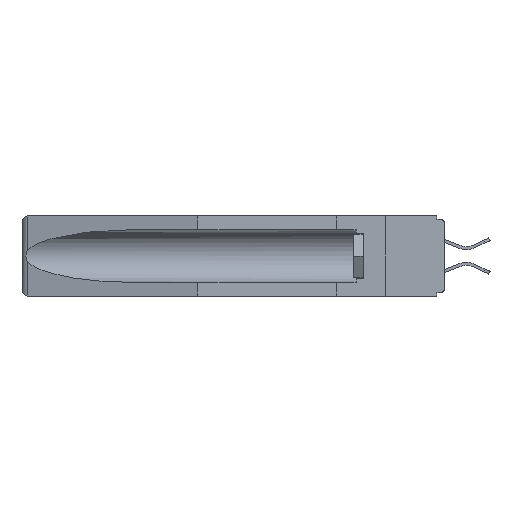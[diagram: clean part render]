
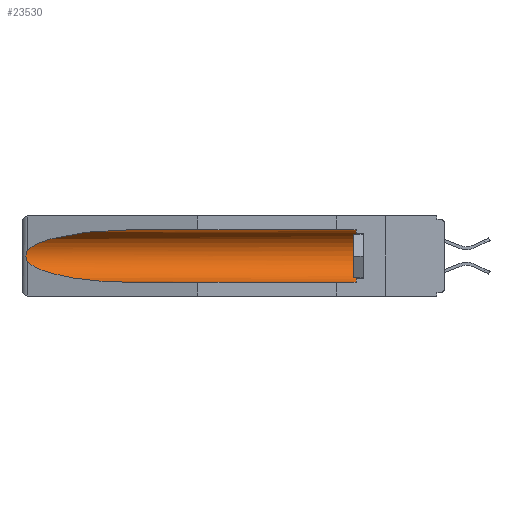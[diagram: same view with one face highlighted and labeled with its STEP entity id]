
A CAD part, left-side view. The second image highlights one B-rep face of the part: STEP entity #23530.
In plain terms, the highlighted cylindrical face has radius 2.857 mm (diameter 5.715 mm), a partial arc.
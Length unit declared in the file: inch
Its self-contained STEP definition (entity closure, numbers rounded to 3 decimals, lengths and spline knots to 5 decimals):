
#52 = DIRECTION ( 'NONE',  ( 0., 0., 1. ) ) ;
#1085 = VERTEX_POINT ( 'NONE', #6895 ) ;
#1866 = CARTESIAN_POINT ( 'NONE',  ( 0.155, 1.07973, -0.059 ) ) ;
#2327 = CARTESIAN_POINT ( 'NONE',  ( 0.2675, 1.53308, -0.17534 ) ) ;
#3081 = CARTESIAN_POINT ( 'NONE',  ( 0.26537, 1.52718, -0.14972 ) ) ;
#4478 = CARTESIAN_POINT ( 'NONE',  ( 0.21114, 1.30732, -0.059 ) ) ;
#4778 = LINE ( 'NONE', #22943, #26740 ) ;
#5231 = ORIENTED_EDGE ( 'NONE', *, *, #8693, .T. ) ;
#5910 = CARTESIAN_POINT ( 'NONE',  ( 0.26537, 1.52718, -0.14972 ) ) ;
#6361 = ORIENTED_EDGE ( 'NONE', *, *, #7550, .F. ) ;
#6895 = CARTESIAN_POINT ( 'NONE',  ( 0.155, 0.126, -0.284 ) ) ;
#7322 = DIRECTION ( 'NONE',  ( 0., -1., 0. ) ) ;
#7347 = CARTESIAN_POINT ( 'NONE',  ( 0.26537, 1.52718, -0.19328 ) ) ;
#7550 = EDGE_CURVE ( 'NONE', #1085, #33458, #25398, .T. ) ;
#8027 = CARTESIAN_POINT ( 'NONE',  ( 0.155, 1.07973, -0.284 ) ) ;
#8248 = CARTESIAN_POINT ( 'NONE',  ( 0.155, -0.30754, -0.1715 ) ) ;
#8582 = ORIENTED_EDGE ( 'NONE', *, *, #8944, .T. ) ;
#8693 = EDGE_CURVE ( 'NONE', #29670, #9239, #23338, .T. ) ;
#8930 = CARTESIAN_POINT ( 'NONE',  ( 0.21114, 1.30732, -0.284 ) ) ;
#8944 = EDGE_CURVE ( 'NONE', #17884, #33458, #21247, .T. ) ;
#9044 = CARTESIAN_POINT ( 'NONE',  ( 0.25451, 1.48313, -0.24835 ) ) ;
#9144 = EDGE_CURVE ( 'NONE', #1085, #13082, #14642, .T. ) ;
#9194 = B_SPLINE_CURVE_WITH_KNOTS ( 'NONE', 3,
 ( #25549, #17836, #28146, #22762, #15368, #2327, #33280, #22879, #20251, #7347 ),
 .UNSPECIFIED., .F., .F.,
 ( 4, 2, 2, 2, 4 ),
 ( 0., 0.00029, 0.00058, 0.00087, 0.00117 ),
 .UNSPECIFIED. ) ;
#9239 = VERTEX_POINT ( 'NONE', #5910 ) ;
#9697 = DIRECTION ( 'NONE',  ( 0., 1., 0. ) ) ;
#12210 = AXIS2_PLACEMENT_3D ( 'NONE', #14902, #7322, #28242 ) ;
#13082 = VERTEX_POINT ( 'NONE', #18282 ) ;
#13324 = CARTESIAN_POINT ( 'NONE',  ( 0.26537, 1.52718, -0.19328 ) ) ;
#13930 = EDGE_LOOP ( 'NONE', ( #5231, #24977, #8582, #6361, #14669, #17929 ) ) ;
#14642 = CIRCLE ( 'NONE', #12210, 0.1125 ) ;
#14669 = ORIENTED_EDGE ( 'NONE', *, *, #9144, .T. ) ;
#14902 = CARTESIAN_POINT ( 'NONE',  ( 0.155, 0.126, -0.1715 ) ) ;
#15368 = CARTESIAN_POINT ( 'NONE',  ( 0.2675, 1.53308, -0.16763 ) ) ;
#15626 = DIRECTION ( 'NONE',  ( 0., 1., 0. ) ) ;
#15859 = CARTESIAN_POINT ( 'NONE',  ( 0.155, -0.30754, -0.284 ) ) ;
#17167 = CARTESIAN_POINT ( 'NONE',  ( 0.155, 1.07973, -0.059 ) ) ;
#17569 = VECTOR ( 'NONE', #21223, 39.37008 ) ;
#17774 = CARTESIAN_POINT ( 'NONE',  ( 0.26537, 1.52718, -0.19328 ) ) ;
#17836 = CARTESIAN_POINT ( 'NONE',  ( 0.26597, 1.52961, -0.15275 ) ) ;
#17884 = VERTEX_POINT ( 'NONE', #17774 ) ;
#17929 = ORIENTED_EDGE ( 'NONE', *, *, #24945, .T. ) ;
#18029 = CARTESIAN_POINT ( 'NONE',  ( 0.25451, 1.48313, -0.09465 ) ) ;
#18282 = CARTESIAN_POINT ( 'NONE',  ( 0.155, 0.126, -0.059 ) ) ;
#19483 = CYLINDRICAL_SURFACE ( 'NONE', #28764, 0.1125 ) ;
#20251 = CARTESIAN_POINT ( 'NONE',  ( 0.26597, 1.5296, -0.19026 ) ) ;
#21171 = CARTESIAN_POINT ( 'NONE',  ( 0.155, 1.07973, -0.284 ) ) ;
#21223 = DIRECTION ( 'NONE',  ( 0., 1., 0. ) ) ;
#21247 =( BOUNDED_CURVE ( )  B_SPLINE_CURVE ( 3, ( #13324, #9044, #8930, #21171 ),
 .UNSPECIFIED., .F., .F. ) 
 B_SPLINE_CURVE_WITH_KNOTS ( ( 4, 4 ),
 ( 0.1948, 1.5708 ),
 .UNSPECIFIED. ) 
 CURVE ( )  GEOMETRIC_REPRESENTATION_ITEM ( )  RATIONAL_B_SPLINE_CURVE ( ( 1., 0.848, 0.848, 1. ) ) 
 REPRESENTATION_ITEM ( '' )  );
#22762 = CARTESIAN_POINT ( 'NONE',  ( 0.2673, 1.5327, -0.16383 ) ) ;
#22776 = FACE_OUTER_BOUND ( 'NONE', #13930, .T. ) ;
#22879 = CARTESIAN_POINT ( 'NONE',  ( 0.26655, 1.53094, -0.18657 ) ) ;
#22943 = CARTESIAN_POINT ( 'NONE',  ( 0.155, -0.30754, -0.059 ) ) ;
#23338 =( BOUNDED_CURVE ( )  B_SPLINE_CURVE ( 3, ( #1866, #4478, #18029, #3081 ),
 .UNSPECIFIED., .F., .F. ) 
 B_SPLINE_CURVE_WITH_KNOTS ( ( 4, 4 ),
 ( 4.71239, 6.08839 ),
 .UNSPECIFIED. ) 
 CURVE ( )  GEOMETRIC_REPRESENTATION_ITEM ( )  RATIONAL_B_SPLINE_CURVE ( ( 1., 0.848, 0.848, 1. ) ) 
 REPRESENTATION_ITEM ( '' )  );
#23530 = ADVANCED_FACE ( 'NONE', ( #22776 ), #19483, .F. ) ;
#24945 = EDGE_CURVE ( 'NONE', #13082, #29670, #4778, .T. ) ;
#24977 = ORIENTED_EDGE ( 'NONE', *, *, #28274, .T. ) ;
#25398 = LINE ( 'NONE', #15859, #17569 ) ;
#25549 = CARTESIAN_POINT ( 'NONE',  ( 0.26537, 1.52718, -0.14972 ) ) ;
#26740 = VECTOR ( 'NONE', #9697, 39.37008 ) ;
#28146 = CARTESIAN_POINT ( 'NONE',  ( 0.26654, 1.53092, -0.15636 ) ) ;
#28242 = DIRECTION ( 'NONE',  ( 0., 0., 1. ) ) ;
#28274 = EDGE_CURVE ( 'NONE', #9239, #17884, #9194, .T. ) ;
#28764 = AXIS2_PLACEMENT_3D ( 'NONE', #8248, #15626, #52 ) ;
#29670 = VERTEX_POINT ( 'NONE', #17167 ) ;
#33280 = CARTESIAN_POINT ( 'NONE',  ( 0.2673, 1.53269, -0.17917 ) ) ;
#33458 = VERTEX_POINT ( 'NONE', #8027 ) ;
